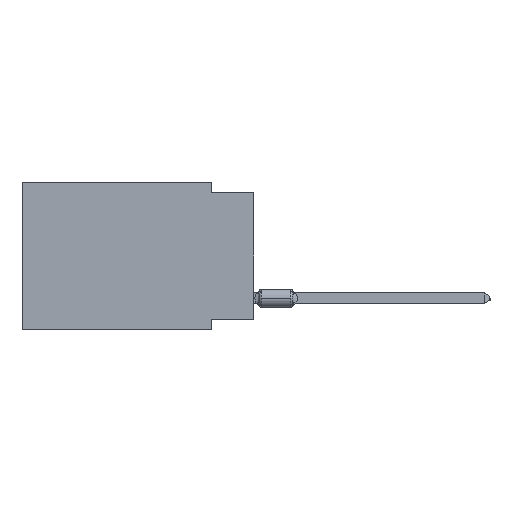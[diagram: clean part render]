
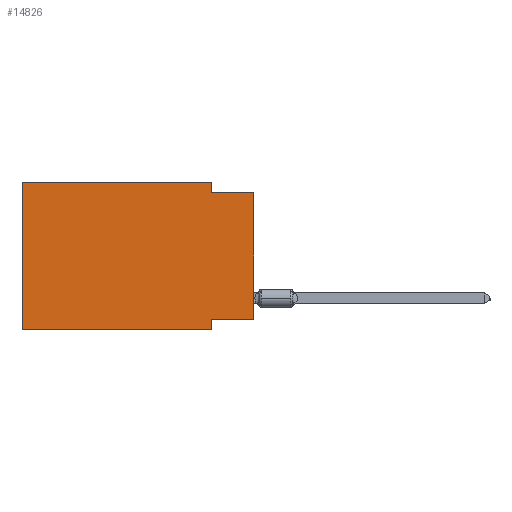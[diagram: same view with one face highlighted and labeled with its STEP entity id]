
A CAD part, left-side view. The second image highlights one B-rep face of the part: STEP entity #14826.
In plain terms, the highlighted planar face has unit normal (-1, 0, 0).
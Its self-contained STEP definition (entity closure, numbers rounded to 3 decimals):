
#58 = CARTESIAN_POINT ( 'NONE',  ( 0., 0., 0. ) ) ;
#642 = VECTOR ( 'NONE', #1726, 1000. ) ;
#1726 = DIRECTION ( 'NONE',  ( 0., 0., 1. ) ) ;
#1784 = CARTESIAN_POINT ( 'NONE',  ( 0., 2.54, -8.89 ) ) ;
#2116 = EDGE_CURVE ( 'NONE', #34033, #8764, #39361, .T. ) ;
#3012 = VECTOR ( 'NONE', #36567, 1000. ) ;
#5210 = DIRECTION ( 'NONE',  ( 0., 0., 1. ) ) ;
#5323 = LINE ( 'NONE', #37997, #49276 ) ;
#5920 = CARTESIAN_POINT ( 'NONE',  ( 0., 2.54, -0.635 ) ) ;
#7425 = FACE_OUTER_BOUND ( 'NONE', #29859, .T. ) ;
#8764 = VERTEX_POINT ( 'NONE', #20173 ) ;
#10325 = VECTOR ( 'NONE', #48444, 1000. ) ;
#10861 = ORIENTED_EDGE ( 'NONE', *, *, #16762, .F. ) ;
#11398 = ORIENTED_EDGE ( 'NONE', *, *, #25685, .F. ) ;
#11945 = CARTESIAN_POINT ( 'NONE',  ( 0., 13.97, 0. ) ) ;
#12060 = ORIENTED_EDGE ( 'NONE', *, *, #50004, .T. ) ;
#12736 = CARTESIAN_POINT ( 'NONE',  ( 0., 13.97, 0. ) ) ;
#14343 = DIRECTION ( 'NONE',  ( 0., 0., -1. ) ) ;
#14826 = ADVANCED_FACE ( 'NONE', ( #7425 ), #44325, .F. ) ;
#16762 = EDGE_CURVE ( 'NONE', #36224, #52764, #27947, .T. ) ;
#17465 = VERTEX_POINT ( 'NONE', #46497 ) ;
#20010 = DIRECTION ( 'NONE',  ( 0., 1., 0. ) ) ;
#20173 = CARTESIAN_POINT ( 'NONE',  ( 0., 2.54, -8.255 ) ) ;
#21319 = DIRECTION ( 'NONE',  ( 0., 0., -1. ) ) ;
#25408 = CARTESIAN_POINT ( 'NONE',  ( 0., 0., -8.255 ) ) ;
#25685 = EDGE_CURVE ( 'NONE', #52764, #46659, #46251, .T. ) ;
#27947 = LINE ( 'NONE', #55799, #45848 ) ;
#28489 = LINE ( 'NONE', #58, #36890 ) ;
#29314 = LINE ( 'NONE', #1784, #37765 ) ;
#29859 = EDGE_LOOP ( 'NONE', ( #12060, #11398, #10861, #31842, #44963, #35222, #53130, #57360 ) ) ;
#29994 = CARTESIAN_POINT ( 'NONE',  ( 0., 13.97, -8.89 ) ) ;
#30265 = CARTESIAN_POINT ( 'NONE',  ( 0., 0., -8.255 ) ) ;
#31842 = ORIENTED_EDGE ( 'NONE', *, *, #37006, .F. ) ;
#32159 = VECTOR ( 'NONE', #20010, 1000. ) ;
#33605 = CARTESIAN_POINT ( 'NONE',  ( 0., 2.54, 0. ) ) ;
#34033 = VERTEX_POINT ( 'NONE', #25408 ) ;
#34098 = CARTESIAN_POINT ( 'NONE',  ( 0., 13.97, 0. ) ) ;
#35222 = ORIENTED_EDGE ( 'NONE', *, *, #57708, .T. ) ;
#36224 = VERTEX_POINT ( 'NONE', #33605 ) ;
#36567 = DIRECTION ( 'NONE',  ( 0., -1., 0. ) ) ;
#36852 = AXIS2_PLACEMENT_3D ( 'NONE', #11945, #58832, #21319 ) ;
#36890 = VECTOR ( 'NONE', #5210, 1000. ) ;
#37006 = EDGE_CURVE ( 'NONE', #45767, #36224, #5323, .T. ) ;
#37482 = CARTESIAN_POINT ( 'NONE',  ( 0., 0., -0.635 ) ) ;
#37765 = VECTOR ( 'NONE', #52024, 1000. ) ;
#37997 = CARTESIAN_POINT ( 'NONE',  ( 0., 13.97, 0. ) ) ;
#39361 = LINE ( 'NONE', #30265, #32159 ) ;
#41657 = CARTESIAN_POINT ( 'NONE',  ( 0., 0., -0.635 ) ) ;
#42642 = VERTEX_POINT ( 'NONE', #48109 ) ;
#44325 = PLANE ( 'NONE',  #36852 ) ;
#44963 = ORIENTED_EDGE ( 'NONE', *, *, #56161, .F. ) ;
#45767 = VERTEX_POINT ( 'NONE', #12736 ) ;
#45848 = VECTOR ( 'NONE', #14343, 1000. ) ;
#46251 = LINE ( 'NONE', #37482, #3012 ) ;
#46497 = CARTESIAN_POINT ( 'NONE',  ( 0., 2.54, -8.89 ) ) ;
#46659 = VERTEX_POINT ( 'NONE', #41657 ) ;
#48109 = CARTESIAN_POINT ( 'NONE',  ( 0., 13.97, -8.89 ) ) ;
#48296 = LINE ( 'NONE', #34098, #642 ) ;
#48444 = DIRECTION ( 'NONE',  ( 0., -1., 0. ) ) ;
#49276 = VECTOR ( 'NONE', #56435, 1000. ) ;
#50004 = EDGE_CURVE ( 'NONE', #34033, #46659, #28489, .T. ) ;
#50566 = EDGE_CURVE ( 'NONE', #8764, #17465, #29314, .T. ) ;
#52024 = DIRECTION ( 'NONE',  ( 0., 0., -1. ) ) ;
#52764 = VERTEX_POINT ( 'NONE', #5920 ) ;
#52990 = LINE ( 'NONE', #29994, #10325 ) ;
#53130 = ORIENTED_EDGE ( 'NONE', *, *, #50566, .F. ) ;
#55799 = CARTESIAN_POINT ( 'NONE',  ( 0., 2.54, 0. ) ) ;
#56161 = EDGE_CURVE ( 'NONE', #42642, #45767, #48296, .T. ) ;
#56435 = DIRECTION ( 'NONE',  ( 0., -1., 0. ) ) ;
#57360 = ORIENTED_EDGE ( 'NONE', *, *, #2116, .F. ) ;
#57708 = EDGE_CURVE ( 'NONE', #42642, #17465, #52990, .T. ) ;
#58832 = DIRECTION ( 'NONE',  ( 1., 0., 0. ) ) ;
